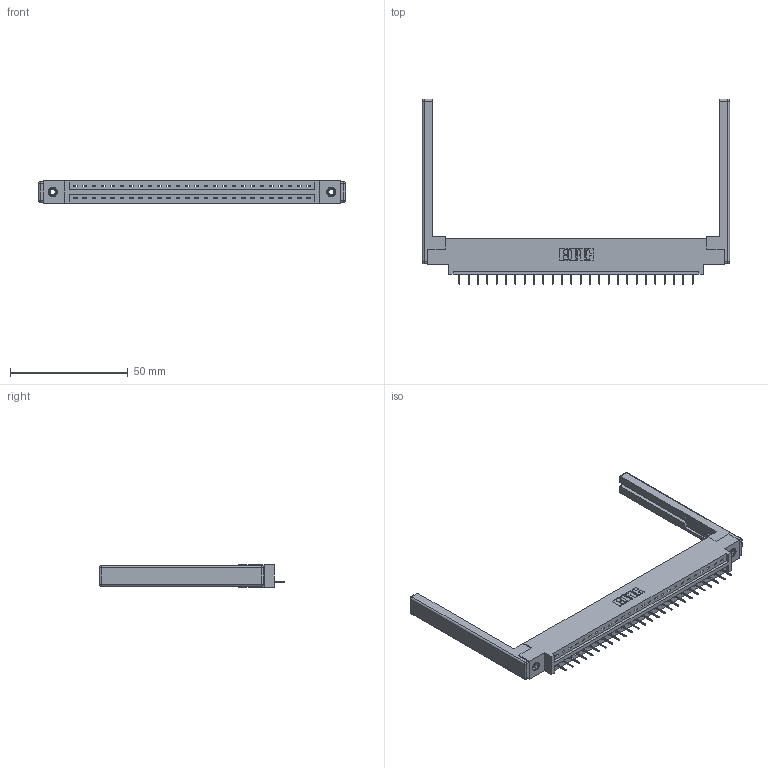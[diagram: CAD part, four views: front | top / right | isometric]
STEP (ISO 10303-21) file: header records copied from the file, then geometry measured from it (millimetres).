
FILE_DESCRIPTION (( 'STEP AP203' ), '1' );
FILE_NAME ('387-026-524-668.STEP', '2019-10-03T12:39:31', ( '' ), ( '' ), 'SwSTEP 2.0', 'SolidWorks 2016', '' );
FILE_SCHEMA (( 'CONFIG_CONTROL_DESIGN' ));
Length unit declared in the file: inch
Products named in the file (5): 337 Part_0.170 Offset - 0.156 Dia-TI; 307-220-068; 345-250-001_345-250-001-102; 345-292-001_345-293-124; 387-026-524-668
Assembly tree (31 placements, depth 2):
  387-026-524-668
    337 Part_0.170 Offset - 0.156 Dia-TI
    345-292-001_345-293-124  x26
    345-250-001_345-250-001-102  x2
    307-220-068  x2
Bounding box: 130.45 x 78.75 x 9.4 mm (x, y, z)
Volume: 17529.3 mm3; surface area: 17315.4 mm2
Topology: 31 solids, 31 shells, 1988 faces, 5705 edges, 3678 vertices
Faces by surface type: plane 1514, cylinder 450, cone 12, sphere 8, torus 4
Entity records: 24362 total; most frequent: CARTESIAN_POINT 4197, ORIENTED_EDGE 4148, DIRECTION 3640, EDGE_CURVE 2074, VECTOR 1900, LINE 1900, VERTEX_POINT 1370, AXIS2_PLACEMENT_3D 870
